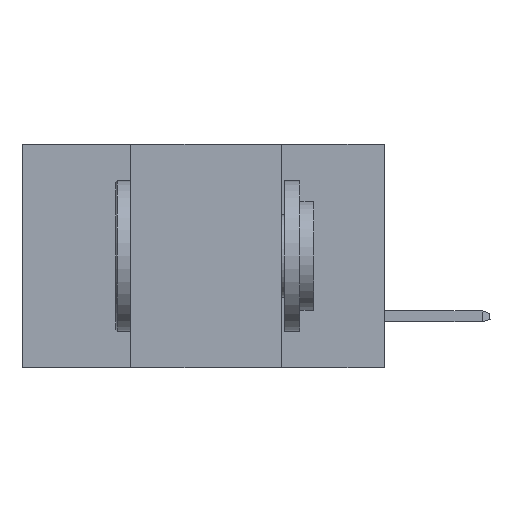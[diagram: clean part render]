
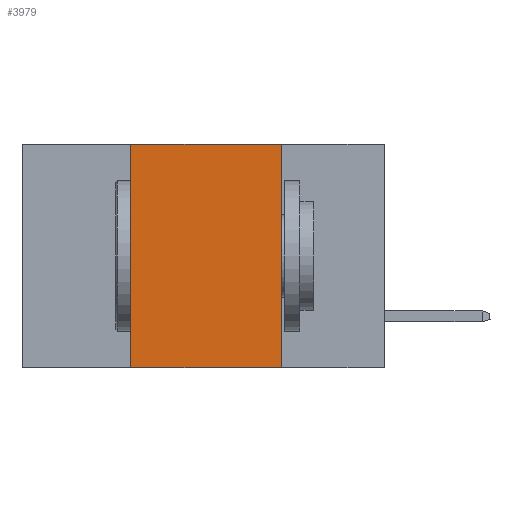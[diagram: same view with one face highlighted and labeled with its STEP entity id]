
A CAD part, left-side view. The second image highlights one B-rep face of the part: STEP entity #3979.
In plain terms, the highlighted planar face has unit normal (-1, 0, 0).
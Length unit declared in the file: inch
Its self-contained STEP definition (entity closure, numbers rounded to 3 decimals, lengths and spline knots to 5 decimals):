
#72 = ORIENTED_EDGE ( 'NONE', *, *, #10303, .F. ) ;
#664 = FACE_OUTER_BOUND ( 'NONE', #9793, .T. ) ;
#1217 = CARTESIAN_POINT ( 'NONE',  ( 0., 0.6, -0.37 ) ) ;
#1249 = DIRECTION ( 'NONE',  ( 0., -1., 0. ) ) ;
#1311 = LINE ( 'NONE', #8988, #7613 ) ;
#1818 = CARTESIAN_POINT ( 'NONE',  ( 0., 0.6, 0. ) ) ;
#1986 = CARTESIAN_POINT ( 'NONE',  ( 0., 0.42, 0. ) ) ;
#2052 = CARTESIAN_POINT ( 'NONE',  ( 0., 0.17, 0. ) ) ;
#2336 = CARTESIAN_POINT ( 'NONE',  ( 0., 0.42, -0.37 ) ) ;
#2501 = VERTEX_POINT ( 'NONE', #3384 ) ;
#2887 = AXIS2_PLACEMENT_3D ( 'NONE', #3547, #10147, #5308 ) ;
#2892 = VECTOR ( 'NONE', #7586, 39.37008 ) ;
#2906 = VECTOR ( 'NONE', #1249, 39.37008 ) ;
#2916 = DIRECTION ( 'NONE',  ( 0., 0., -1. ) ) ;
#3384 = CARTESIAN_POINT ( 'NONE',  ( 0., 0.17, -0.37 ) ) ;
#3547 = CARTESIAN_POINT ( 'NONE',  ( 0., 0.6, 0. ) ) ;
#3696 = PLANE ( 'NONE',  #2887 ) ;
#3927 = ORIENTED_EDGE ( 'NONE', *, *, #4275, .F. ) ;
#3979 = ADVANCED_FACE ( 'NONE', ( #664 ), #3696, .F. ) ;
#4275 = EDGE_CURVE ( 'NONE', #9709, #4514, #1311, .T. ) ;
#4514 = VERTEX_POINT ( 'NONE', #1986 ) ;
#4887 = VECTOR ( 'NONE', #2916, 39.37008 ) ;
#5308 = DIRECTION ( 'NONE',  ( 0., 0., -1. ) ) ;
#5832 = LINE ( 'NONE', #1818, #2892 ) ;
#6334 = EDGE_CURVE ( 'NONE', #9709, #2501, #6345, .T. ) ;
#6345 = LINE ( 'NONE', #1217, #2906 ) ;
#6570 = EDGE_CURVE ( 'NONE', #8249, #2501, #9242, .T. ) ;
#7032 = ORIENTED_EDGE ( 'NONE', *, *, #6334, .T. ) ;
#7586 = DIRECTION ( 'NONE',  ( 0., -1., 0. ) ) ;
#7613 = VECTOR ( 'NONE', #9875, 39.37008 ) ;
#7730 = CARTESIAN_POINT ( 'NONE',  ( 0., 0.17, 0. ) ) ;
#8249 = VERTEX_POINT ( 'NONE', #2052 ) ;
#8988 = CARTESIAN_POINT ( 'NONE',  ( 0., 0.42, 0. ) ) ;
#9242 = LINE ( 'NONE', #7730, #4887 ) ;
#9431 = ORIENTED_EDGE ( 'NONE', *, *, #6570, .F. ) ;
#9709 = VERTEX_POINT ( 'NONE', #2336 ) ;
#9793 = EDGE_LOOP ( 'NONE', ( #9431, #72, #3927, #7032 ) ) ;
#9875 = DIRECTION ( 'NONE',  ( 0., 0., 1. ) ) ;
#10147 = DIRECTION ( 'NONE',  ( 1., 0., 0. ) ) ;
#10303 = EDGE_CURVE ( 'NONE', #4514, #8249, #5832, .T. ) ;
